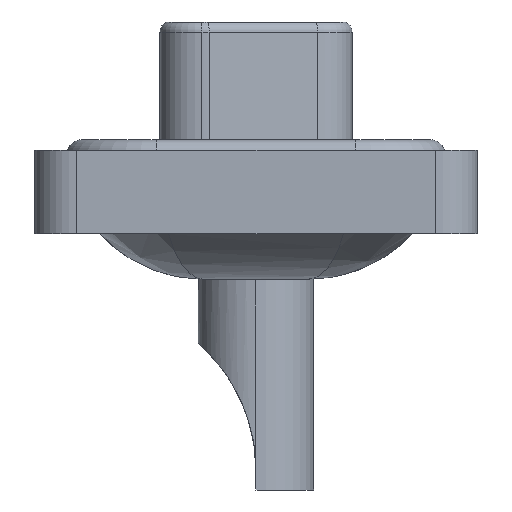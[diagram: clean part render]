
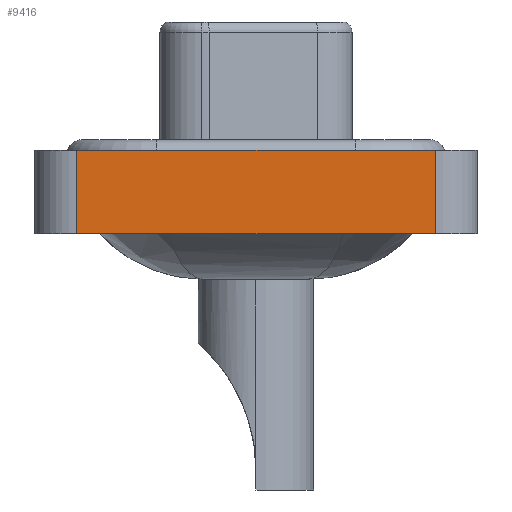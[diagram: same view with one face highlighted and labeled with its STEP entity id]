
A CAD part, left-side view. The second image highlights one B-rep face of the part: STEP entity #9416.
In plain terms, the highlighted planar face has unit normal (-1, 0, 0).
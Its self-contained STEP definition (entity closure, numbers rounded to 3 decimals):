
#1073 = CARTESIAN_POINT ( 'NONE',  ( -7.25, -8.55, -3.6 ) ) ;
#1199 = VERTEX_POINT ( 'NONE', #7182 ) ;
#1986 = VERTEX_POINT ( 'NONE', #15012 ) ;
#2946 = EDGE_CURVE ( 'NONE', #13049, #10347, #3091, .T. ) ;
#3012 = CARTESIAN_POINT ( 'NONE',  ( -7.25, -8.55, -3.6 ) ) ;
#3091 = LINE ( 'NONE', #7712, #14461 ) ;
#3316 = ORIENTED_EDGE ( 'NONE', *, *, #10710, .T. ) ;
#3476 = CARTESIAN_POINT ( 'NONE',  ( -7.25, -8.55, -3.6 ) ) ;
#4309 = ORIENTED_EDGE ( 'NONE', *, *, #2946, .T. ) ;
#5539 = CARTESIAN_POINT ( 'NONE',  ( -7.25, -8.55, 0.4 ) ) ;
#6915 = EDGE_CURVE ( 'NONE', #1986, #1199, #10921, .T. ) ;
#7182 = CARTESIAN_POINT ( 'NONE',  ( -7.25, 8.55, 0.4 ) ) ;
#7494 = LINE ( 'NONE', #16203, #14786 ) ;
#7689 = EDGE_CURVE ( 'NONE', #1199, #10347, #7494, .T. ) ;
#7712 = CARTESIAN_POINT ( 'NONE',  ( -7.25, -8.55, -3.6 ) ) ;
#8576 = AXIS2_PLACEMENT_3D ( 'NONE', #3476, #9139, #16002 ) ;
#9139 = DIRECTION ( 'NONE',  ( -1., 0., 0. ) ) ;
#9416 = ADVANCED_FACE ( 'NONE', ( #16186 ), #13219, .T. ) ;
#9690 = ORIENTED_EDGE ( 'NONE', *, *, #6915, .F. ) ;
#10347 = VERTEX_POINT ( 'NONE', #5539 ) ;
#10710 = EDGE_CURVE ( 'NONE', #1986, #13049, #16375, .T. ) ;
#10728 = VECTOR ( 'NONE', #12569, 1000. ) ;
#10921 = LINE ( 'NONE', #17595, #14812 ) ;
#11480 = EDGE_LOOP ( 'NONE', ( #4309, #17674, #9690, #3316 ) ) ;
#12569 = DIRECTION ( 'NONE',  ( 0., -1., 0. ) ) ;
#13049 = VERTEX_POINT ( 'NONE', #3012 ) ;
#13151 = DIRECTION ( 'NONE',  ( 0., -1., 0. ) ) ;
#13219 = PLANE ( 'NONE',  #8576 ) ;
#13278 = DIRECTION ( 'NONE',  ( 0., 0., 1. ) ) ;
#14461 = VECTOR ( 'NONE', #13278, 1000. ) ;
#14786 = VECTOR ( 'NONE', #13151, 1000. ) ;
#14812 = VECTOR ( 'NONE', #17771, 1000. ) ;
#15012 = CARTESIAN_POINT ( 'NONE',  ( -7.25, 8.55, -3.6 ) ) ;
#16002 = DIRECTION ( 'NONE',  ( 0., 0., 1. ) ) ;
#16186 = FACE_OUTER_BOUND ( 'NONE', #11480, .T. ) ;
#16203 = CARTESIAN_POINT ( 'NONE',  ( -7.25, -8.55, 0.4 ) ) ;
#16375 = LINE ( 'NONE', #1073, #10728 ) ;
#17595 = CARTESIAN_POINT ( 'NONE',  ( -7.25, 8.55, -3.6 ) ) ;
#17674 = ORIENTED_EDGE ( 'NONE', *, *, #7689, .F. ) ;
#17771 = DIRECTION ( 'NONE',  ( 0., 0., 1. ) ) ;
